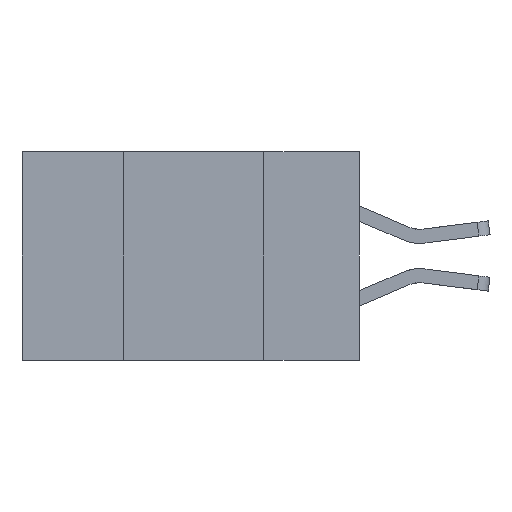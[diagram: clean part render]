
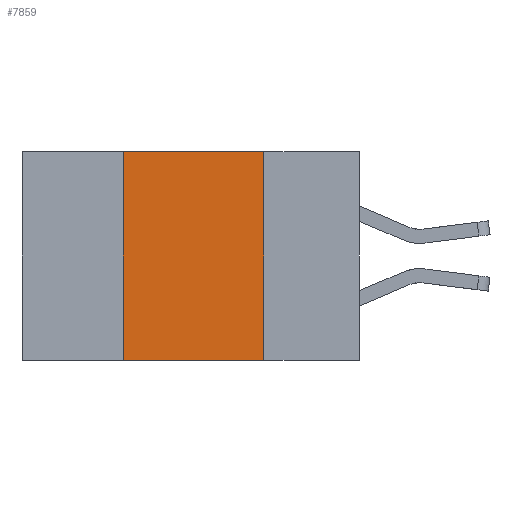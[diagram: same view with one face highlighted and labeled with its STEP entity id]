
A CAD part, left-side view. The second image highlights one B-rep face of the part: STEP entity #7859.
In plain terms, the highlighted planar face has unit normal (-1, 0, 0).
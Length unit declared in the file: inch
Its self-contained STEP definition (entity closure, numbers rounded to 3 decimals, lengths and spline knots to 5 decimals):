
#999 = ORIENTED_EDGE ( 'NONE', *, *, #9332, .F. ) ;
#1049 = VERTEX_POINT ( 'NONE', #7427 ) ;
#1182 = VECTOR ( 'NONE', #3439, 39.37008 ) ;
#1406 = CARTESIAN_POINT ( 'NONE',  ( 0., 0.17, 0. ) ) ;
#2191 = PLANE ( 'NONE',  #7204 ) ;
#2779 = EDGE_LOOP ( 'NONE', ( #7641, #999, #5537, #5701 ) ) ;
#3059 = DIRECTION ( 'NONE',  ( 0., 0., -1. ) ) ;
#3095 = LINE ( 'NONE', #1406, #9865 ) ;
#3439 = DIRECTION ( 'NONE',  ( 0., -1., 0. ) ) ;
#3532 = LINE ( 'NONE', #5304, #1182 ) ;
#4769 = DIRECTION ( 'NONE',  ( 0., 0., 1. ) ) ;
#5255 = VECTOR ( 'NONE', #6327, 39.37008 ) ;
#5304 = CARTESIAN_POINT ( 'NONE',  ( 0., 0.6, -0.37 ) ) ;
#5451 = CARTESIAN_POINT ( 'NONE',  ( 0., 0.6, 0. ) ) ;
#5537 = ORIENTED_EDGE ( 'NONE', *, *, #8702, .F. ) ;
#5658 = VERTEX_POINT ( 'NONE', #7631 ) ;
#5701 = ORIENTED_EDGE ( 'NONE', *, *, #7544, .T. ) ;
#5702 = CARTESIAN_POINT ( 'NONE',  ( 0., 0.42, 0. ) ) ;
#6087 = VECTOR ( 'NONE', #4769, 39.37008 ) ;
#6088 = VERTEX_POINT ( 'NONE', #8644 ) ;
#6327 = DIRECTION ( 'NONE',  ( 0., -1., 0. ) ) ;
#6794 = FACE_OUTER_BOUND ( 'NONE', #2779, .T. ) ;
#7204 = AXIS2_PLACEMENT_3D ( 'NONE', #10838, #8417, #3059 ) ;
#7307 = VERTEX_POINT ( 'NONE', #10158 ) ;
#7427 = CARTESIAN_POINT ( 'NONE',  ( 0., 0.17, 0. ) ) ;
#7544 = EDGE_CURVE ( 'NONE', #7307, #6088, #3532, .T. ) ;
#7625 = LINE ( 'NONE', #5451, #5255 ) ;
#7631 = CARTESIAN_POINT ( 'NONE',  ( 0., 0.42, 0. ) ) ;
#7641 = ORIENTED_EDGE ( 'NONE', *, *, #9823, .F. ) ;
#7701 = DIRECTION ( 'NONE',  ( 0., 0., -1. ) ) ;
#7859 = ADVANCED_FACE ( 'NONE', ( #6794 ), #2191, .F. ) ;
#8417 = DIRECTION ( 'NONE',  ( 1., 0., 0. ) ) ;
#8644 = CARTESIAN_POINT ( 'NONE',  ( 0., 0.17, -0.37 ) ) ;
#8702 = EDGE_CURVE ( 'NONE', #7307, #5658, #10614, .T. ) ;
#9332 = EDGE_CURVE ( 'NONE', #5658, #1049, #7625, .T. ) ;
#9823 = EDGE_CURVE ( 'NONE', #1049, #6088, #3095, .T. ) ;
#9865 = VECTOR ( 'NONE', #7701, 39.37008 ) ;
#10158 = CARTESIAN_POINT ( 'NONE',  ( 0., 0.42, -0.37 ) ) ;
#10614 = LINE ( 'NONE', #5702, #6087 ) ;
#10838 = CARTESIAN_POINT ( 'NONE',  ( 0., 0.6, 0. ) ) ;
